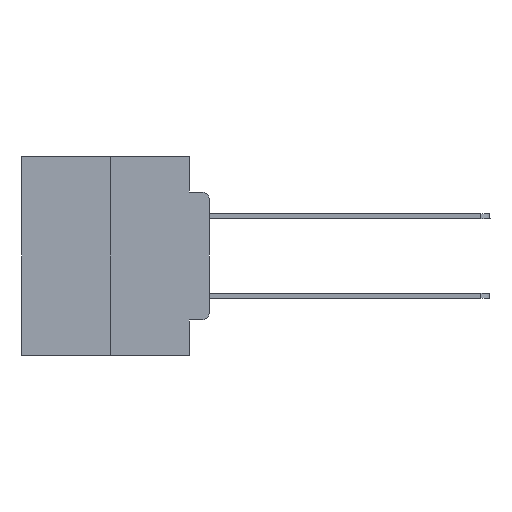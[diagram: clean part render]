
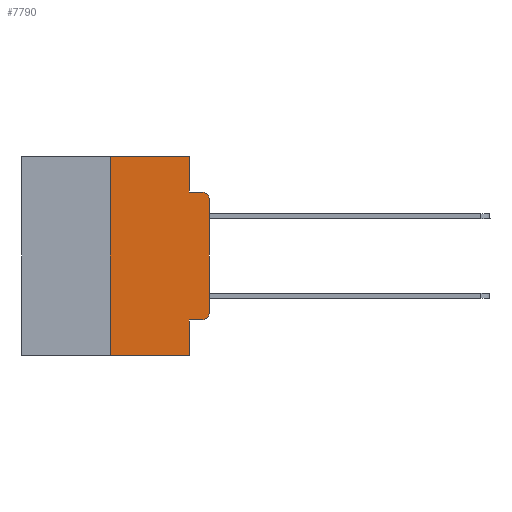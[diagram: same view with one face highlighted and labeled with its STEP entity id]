
A CAD part, left-side view. The second image highlights one B-rep face of the part: STEP entity #7790.
In plain terms, the highlighted planar face has unit normal (-1, 0, 0).
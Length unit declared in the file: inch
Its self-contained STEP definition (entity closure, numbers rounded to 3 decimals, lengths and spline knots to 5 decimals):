
#24 = VERTEX_POINT ( 'NONE', #25526 ) ;
#69 = LINE ( 'NONE', #2450, #16126 ) ;
#99 = EDGE_CURVE ( 'NONE', #24, #3620, #749, .T. ) ;
#618 = CARTESIAN_POINT ( 'NONE',  ( 0., 0.02, -0.0885 ) ) ;
#749 = LINE ( 'NONE', #17785, #16481 ) ;
#784 = EDGE_CURVE ( 'NONE', #3989, #20879, #69, .T. ) ;
#1022 = EDGE_CURVE ( 'NONE', #12394, #2336, #19659, .T. ) ;
#1426 = CARTESIAN_POINT ( 'NONE',  ( 0., 0.25, 0. ) ) ;
#1472 = CARTESIAN_POINT ( 'NONE',  ( 0., 0., 0. ) ) ;
#1510 = ORIENTED_EDGE ( 'NONE', *, *, #5814, .F. ) ;
#2277 = CIRCLE ( 'NONE', #24474, 0.02 ) ;
#2336 = VERTEX_POINT ( 'NONE', #618 ) ;
#2450 = CARTESIAN_POINT ( 'NONE',  ( 0., 0.25, 0. ) ) ;
#2480 = FACE_OUTER_BOUND ( 'NONE', #26530, .T. ) ;
#2846 = VERTEX_POINT ( 'NONE', #25654 ) ;
#3336 = DIRECTION ( 'NONE',  ( 0., 0., -1. ) ) ;
#3395 = CARTESIAN_POINT ( 'NONE',  ( 0., 0.473, -0.5 ) ) ;
#3487 = CARTESIAN_POINT ( 'NONE',  ( 0., 0.473, 0. ) ) ;
#3620 = VERTEX_POINT ( 'NONE', #10202 ) ;
#3981 = AXIS2_PLACEMENT_3D ( 'NONE', #4364, #4094, #22487 ) ;
#3989 = VERTEX_POINT ( 'NONE', #22723 ) ;
#4094 = DIRECTION ( 'NONE',  ( -1., 0., 0. ) ) ;
#4364 = CARTESIAN_POINT ( 'NONE',  ( 0., 0.02, -0.1085 ) ) ;
#5630 = ORIENTED_EDGE ( 'NONE', *, *, #1022, .F. ) ;
#5642 = DIRECTION ( 'NONE',  ( 0., 0., 1. ) ) ;
#5685 = VERTEX_POINT ( 'NONE', #8309 ) ;
#5814 = EDGE_CURVE ( 'NONE', #20879, #2846, #13841, .T. ) ;
#6280 = ORIENTED_EDGE ( 'NONE', *, *, #6333, .T. ) ;
#6333 = EDGE_CURVE ( 'NONE', #22101, #2336, #12848, .T. ) ;
#6686 = LINE ( 'NONE', #7021, #16925 ) ;
#6838 = CARTESIAN_POINT ( 'NONE',  ( 0., 0., -0.3915 ) ) ;
#7021 = CARTESIAN_POINT ( 'NONE',  ( 0., 0.051, -0.4115 ) ) ;
#7095 = LINE ( 'NONE', #3395, #11200 ) ;
#7559 = DIRECTION ( 'NONE',  ( 0., -1., 0. ) ) ;
#7781 = VECTOR ( 'NONE', #8752, 39.37008 ) ;
#7790 = ADVANCED_FACE ( 'NONE', ( #2480 ), #21892, .F. ) ;
#7841 = CARTESIAN_POINT ( 'NONE',  ( 0., 0.02, -0.3915 ) ) ;
#8223 = VECTOR ( 'NONE', #25696, 39.37008 ) ;
#8309 = CARTESIAN_POINT ( 'NONE',  ( 0., 0.02, -0.4115 ) ) ;
#8639 = ORIENTED_EDGE ( 'NONE', *, *, #22835, .T. ) ;
#8752 = DIRECTION ( 'NONE',  ( 0., -1., 0. ) ) ;
#9570 = CARTESIAN_POINT ( 'NONE',  ( 0., 0., -0.1085 ) ) ;
#9708 = VERTEX_POINT ( 'NONE', #6838 ) ;
#10202 = CARTESIAN_POINT ( 'NONE',  ( 0., 0.051, -0.5 ) ) ;
#11034 = VECTOR ( 'NONE', #5642, 39.37008 ) ;
#11200 = VECTOR ( 'NONE', #7559, 39.37008 ) ;
#12394 = VERTEX_POINT ( 'NONE', #15753 ) ;
#12799 = ORIENTED_EDGE ( 'NONE', *, *, #24637, .T. ) ;
#12848 = CIRCLE ( 'NONE', #3981, 0.02 ) ;
#13841 = LINE ( 'NONE', #16800, #7781 ) ;
#13972 = DIRECTION ( 'NONE',  ( -1., 0., 0. ) ) ;
#15149 = ORIENTED_EDGE ( 'NONE', *, *, #18865, .T. ) ;
#15753 = CARTESIAN_POINT ( 'NONE',  ( 0., 0.051, -0.0885 ) ) ;
#15962 = DIRECTION ( 'NONE',  ( 0., 0., -1. ) ) ;
#16126 = VECTOR ( 'NONE', #25705, 39.37008 ) ;
#16210 = ORIENTED_EDGE ( 'NONE', *, *, #16902, .F. ) ;
#16246 = CARTESIAN_POINT ( 'NONE',  ( 0., 0.051, -0.0885 ) ) ;
#16481 = VECTOR ( 'NONE', #3336, 39.37008 ) ;
#16800 = CARTESIAN_POINT ( 'NONE',  ( 0., 0.473, 0. ) ) ;
#16902 = EDGE_CURVE ( 'NONE', #2846, #12394, #22966, .T. ) ;
#16925 = VECTOR ( 'NONE', #21347, 39.37008 ) ;
#17664 = DIRECTION ( 'NONE',  ( 0., 0., -1. ) ) ;
#17777 = LINE ( 'NONE', #1472, #11034 ) ;
#17785 = CARTESIAN_POINT ( 'NONE',  ( 0., 0.051, 0. ) ) ;
#17953 = ORIENTED_EDGE ( 'NONE', *, *, #784, .F. ) ;
#18865 = EDGE_CURVE ( 'NONE', #5685, #9708, #2277, .T. ) ;
#19291 = ORIENTED_EDGE ( 'NONE', *, *, #26470, .T. ) ;
#19659 = LINE ( 'NONE', #16246, #22239 ) ;
#20343 = AXIS2_PLACEMENT_3D ( 'NONE', #3487, #25926, #17664 ) ;
#20879 = VERTEX_POINT ( 'NONE', #1426 ) ;
#21347 = DIRECTION ( 'NONE',  ( 0., -1., 0. ) ) ;
#21863 = ORIENTED_EDGE ( 'NONE', *, *, #99, .F. ) ;
#21892 = PLANE ( 'NONE',  #20343 ) ;
#22101 = VERTEX_POINT ( 'NONE', #9570 ) ;
#22239 = VECTOR ( 'NONE', #22278, 39.37008 ) ;
#22278 = DIRECTION ( 'NONE',  ( 0., -1., 0. ) ) ;
#22487 = DIRECTION ( 'NONE',  ( 0., 0., -1. ) ) ;
#22723 = CARTESIAN_POINT ( 'NONE',  ( 0., 0.25, -0.5 ) ) ;
#22835 = EDGE_CURVE ( 'NONE', #3989, #3620, #7095, .T. ) ;
#22966 = LINE ( 'NONE', #25256, #8223 ) ;
#24474 = AXIS2_PLACEMENT_3D ( 'NONE', #7841, #13972, #15962 ) ;
#24637 = EDGE_CURVE ( 'NONE', #24, #5685, #6686, .T. ) ;
#25256 = CARTESIAN_POINT ( 'NONE',  ( 0., 0.051, 0. ) ) ;
#25526 = CARTESIAN_POINT ( 'NONE',  ( 0., 0.051, -0.4115 ) ) ;
#25654 = CARTESIAN_POINT ( 'NONE',  ( 0., 0.051, 0. ) ) ;
#25696 = DIRECTION ( 'NONE',  ( 0., 0., -1. ) ) ;
#25705 = DIRECTION ( 'NONE',  ( 0., 0., 1. ) ) ;
#25926 = DIRECTION ( 'NONE',  ( 1., 0., 0. ) ) ;
#26470 = EDGE_CURVE ( 'NONE', #9708, #22101, #17777, .T. ) ;
#26530 = EDGE_LOOP ( 'NONE', ( #19291, #6280, #5630, #16210, #1510, #17953, #8639, #21863, #12799, #15149 ) ) ;
